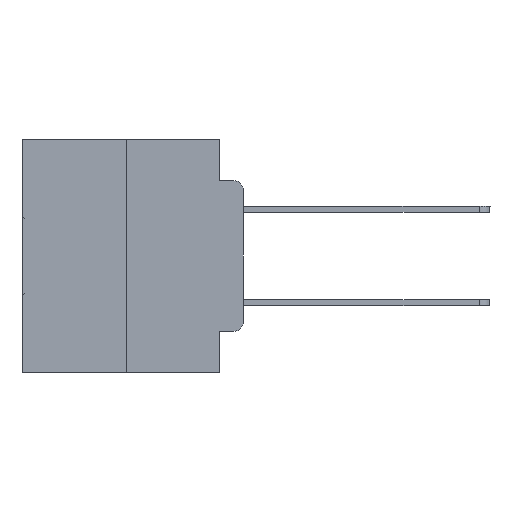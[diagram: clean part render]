
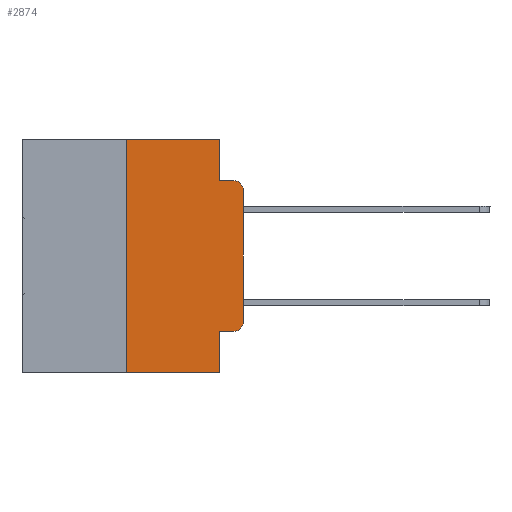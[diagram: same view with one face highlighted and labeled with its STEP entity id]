
A CAD part, left-side view. The second image highlights one B-rep face of the part: STEP entity #2874.
In plain terms, the highlighted planar face has unit normal (-1, 0, 0).
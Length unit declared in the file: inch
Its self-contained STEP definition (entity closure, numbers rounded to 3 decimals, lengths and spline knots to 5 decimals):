
#64 = CARTESIAN_POINT ( 'NONE',  ( 0., 0.02, -0.4115 ) ) ;
#328 = CARTESIAN_POINT ( 'NONE',  ( 0., 0., -0.3915 ) ) ;
#1007 = ORIENTED_EDGE ( 'NONE', *, *, #19235, .T. ) ;
#1326 = VECTOR ( 'NONE', #31915, 39.37008 ) ;
#2069 = VECTOR ( 'NONE', #23760, 39.37008 ) ;
#2664 = DIRECTION ( 'NONE',  ( 0., 0., -1. ) ) ;
#2850 = DIRECTION ( 'NONE',  ( -1., 0., 0. ) ) ;
#2874 = ADVANCED_FACE ( 'NONE', ( #23171 ), #18186, .F. ) ;
#3105 = CARTESIAN_POINT ( 'NONE',  ( 0., 0.051, 0. ) ) ;
#3527 = VECTOR ( 'NONE', #28223, 39.37008 ) ;
#4040 = CIRCLE ( 'NONE', #12324, 0.02 ) ;
#5249 = CARTESIAN_POINT ( 'NONE',  ( 0., 0.051, -0.4115 ) ) ;
#5604 = VERTEX_POINT ( 'NONE', #328 ) ;
#5749 = VERTEX_POINT ( 'NONE', #21079 ) ;
#6037 = CARTESIAN_POINT ( 'NONE',  ( 0., 0.473, 0. ) ) ;
#6176 = VECTOR ( 'NONE', #25906, 39.37008 ) ;
#7036 = LINE ( 'NONE', #16905, #1326 ) ;
#7537 = DIRECTION ( 'NONE',  ( 0., -1., 0. ) ) ;
#7602 = VERTEX_POINT ( 'NONE', #26363 ) ;
#8243 = VECTOR ( 'NONE', #8533, 39.37008 ) ;
#8368 = LINE ( 'NONE', #28403, #3527 ) ;
#8533 = DIRECTION ( 'NONE',  ( 0., -1., 0. ) ) ;
#9843 = LINE ( 'NONE', #19527, #15108 ) ;
#10573 = LINE ( 'NONE', #3105, #6176 ) ;
#10748 = DIRECTION ( 'NONE',  ( 0., 0., -1. ) ) ;
#11275 = CARTESIAN_POINT ( 'NONE',  ( 0., 0.051, -0.0885 ) ) ;
#12061 = AXIS2_PLACEMENT_3D ( 'NONE', #6037, #16090, #10748 ) ;
#12164 = EDGE_CURVE ( 'NONE', #13270, #7602, #8368, .T. ) ;
#12200 = EDGE_CURVE ( 'NONE', #24286, #29530, #20472, .T. ) ;
#12324 = AXIS2_PLACEMENT_3D ( 'NONE', #25698, #13919, #20868 ) ;
#12396 = CARTESIAN_POINT ( 'NONE',  ( 0., 0.25, -0.5 ) ) ;
#12423 = ORIENTED_EDGE ( 'NONE', *, *, #12200, .F. ) ;
#13231 = ORIENTED_EDGE ( 'NONE', *, *, #21218, .T. ) ;
#13270 = VERTEX_POINT ( 'NONE', #12396 ) ;
#13407 = EDGE_CURVE ( 'NONE', #7602, #5749, #17248, .T. ) ;
#13424 = ORIENTED_EDGE ( 'NONE', *, *, #12164, .F. ) ;
#13919 = DIRECTION ( 'NONE',  ( -1., 0., 0. ) ) ;
#14970 = EDGE_CURVE ( 'NONE', #13270, #15334, #7036, .T. ) ;
#15108 = VECTOR ( 'NONE', #2664, 39.37008 ) ;
#15334 = VERTEX_POINT ( 'NONE', #28525 ) ;
#15674 = CARTESIAN_POINT ( 'NONE',  ( 0., 0.051, -0.0885 ) ) ;
#16090 = DIRECTION ( 'NONE',  ( 1., 0., 0. ) ) ;
#16905 = CARTESIAN_POINT ( 'NONE',  ( 0., 0.473, -0.5 ) ) ;
#17236 = ORIENTED_EDGE ( 'NONE', *, *, #24616, .F. ) ;
#17248 = LINE ( 'NONE', #24659, #23517 ) ;
#18186 = PLANE ( 'NONE',  #12061 ) ;
#18893 = EDGE_CURVE ( 'NONE', #30174, #5604, #4040, .T. ) ;
#19078 = LINE ( 'NONE', #23591, #2069 ) ;
#19210 = VERTEX_POINT ( 'NONE', #22438 ) ;
#19235 = EDGE_CURVE ( 'NONE', #24454, #29530, #26276, .T. ) ;
#19527 = CARTESIAN_POINT ( 'NONE',  ( 0., 0.051, 0. ) ) ;
#19711 = DIRECTION ( 'NONE',  ( 0., 0., -1. ) ) ;
#20024 = CARTESIAN_POINT ( 'NONE',  ( 0., 0.02, -0.1085 ) ) ;
#20132 = EDGE_CURVE ( 'NONE', #5749, #24286, #10573, .T. ) ;
#20472 = LINE ( 'NONE', #11275, #8243 ) ;
#20868 = DIRECTION ( 'NONE',  ( 0., 0., -1. ) ) ;
#21079 = CARTESIAN_POINT ( 'NONE',  ( 0., 0.051, 0. ) ) ;
#21218 = EDGE_CURVE ( 'NONE', #5604, #24454, #19078, .T. ) ;
#21638 = CARTESIAN_POINT ( 'NONE',  ( 0., 0., -0.1085 ) ) ;
#22244 = LINE ( 'NONE', #5249, #31220 ) ;
#22429 = ORIENTED_EDGE ( 'NONE', *, *, #20132, .F. ) ;
#22438 = CARTESIAN_POINT ( 'NONE',  ( 0., 0.051, -0.4115 ) ) ;
#22586 = ORIENTED_EDGE ( 'NONE', *, *, #14970, .T. ) ;
#23046 = ORIENTED_EDGE ( 'NONE', *, *, #18893, .T. ) ;
#23171 = FACE_OUTER_BOUND ( 'NONE', #24830, .T. ) ;
#23517 = VECTOR ( 'NONE', #7537, 39.37008 ) ;
#23591 = CARTESIAN_POINT ( 'NONE',  ( 0., 0., 0. ) ) ;
#23760 = DIRECTION ( 'NONE',  ( 0., 0., 1. ) ) ;
#24286 = VERTEX_POINT ( 'NONE', #15674 ) ;
#24454 = VERTEX_POINT ( 'NONE', #21638 ) ;
#24616 = EDGE_CURVE ( 'NONE', #19210, #15334, #9843, .T. ) ;
#24659 = CARTESIAN_POINT ( 'NONE',  ( 0., 0.473, 0. ) ) ;
#24830 = EDGE_LOOP ( 'NONE', ( #13231, #1007, #12423, #22429, #30357, #13424, #22586, #17236, #26457, #23046 ) ) ;
#25698 = CARTESIAN_POINT ( 'NONE',  ( 0., 0.02, -0.3915 ) ) ;
#25906 = DIRECTION ( 'NONE',  ( 0., 0., -1. ) ) ;
#25942 = EDGE_CURVE ( 'NONE', #19210, #30174, #22244, .T. ) ;
#26276 = CIRCLE ( 'NONE', #27290, 0.02 ) ;
#26363 = CARTESIAN_POINT ( 'NONE',  ( 0., 0.25, 0. ) ) ;
#26457 = ORIENTED_EDGE ( 'NONE', *, *, #25942, .T. ) ;
#27290 = AXIS2_PLACEMENT_3D ( 'NONE', #20024, #2850, #19711 ) ;
#28223 = DIRECTION ( 'NONE',  ( 0., 0., 1. ) ) ;
#28403 = CARTESIAN_POINT ( 'NONE',  ( 0., 0.25, 0. ) ) ;
#28525 = CARTESIAN_POINT ( 'NONE',  ( 0., 0.051, -0.5 ) ) ;
#28794 = CARTESIAN_POINT ( 'NONE',  ( 0., 0.02, -0.0885 ) ) ;
#29530 = VERTEX_POINT ( 'NONE', #28794 ) ;
#29536 = DIRECTION ( 'NONE',  ( 0., -1., 0. ) ) ;
#30174 = VERTEX_POINT ( 'NONE', #64 ) ;
#30357 = ORIENTED_EDGE ( 'NONE', *, *, #13407, .F. ) ;
#31220 = VECTOR ( 'NONE', #29536, 39.37008 ) ;
#31915 = DIRECTION ( 'NONE',  ( 0., -1., 0. ) ) ;
